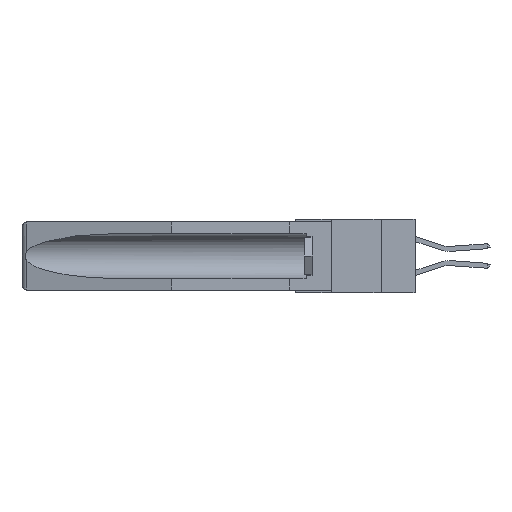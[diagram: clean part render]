
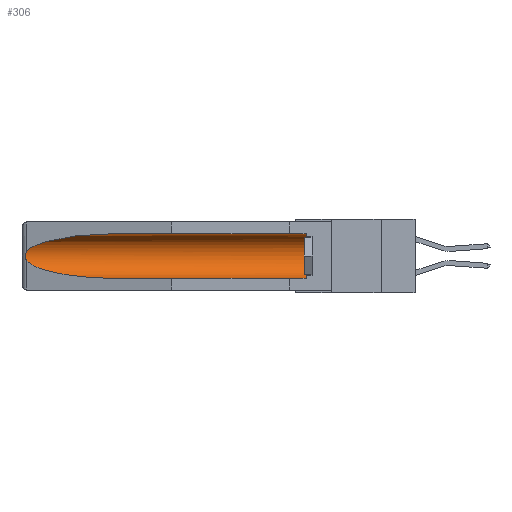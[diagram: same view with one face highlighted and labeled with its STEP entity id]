
A CAD part, left-side view. The second image highlights one B-rep face of the part: STEP entity #306.
In plain terms, the highlighted cylindrical face has radius 2.857 mm (diameter 5.715 mm), a partial arc.
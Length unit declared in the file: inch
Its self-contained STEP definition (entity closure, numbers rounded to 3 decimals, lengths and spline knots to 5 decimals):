
#306 = ADVANCED_FACE ( 'NONE', ( #12683 ), #20967, .F. ) ;
#672 = CARTESIAN_POINT ( 'NONE',  ( 0.26654, 1.53092, -0.15636 ) ) ;
#1336 = CARTESIAN_POINT ( 'NONE',  ( 0.155, 0.126, -0.059 ) ) ;
#1991 = ORIENTED_EDGE ( 'NONE', *, *, #8486, .T. ) ;
#2003 = CARTESIAN_POINT ( 'NONE',  ( 0.155, 0.126, -0.284 ) ) ;
#2503 = CARTESIAN_POINT ( 'NONE',  ( 0.26537, 1.52718, -0.19328 ) ) ;
#3495 = DIRECTION ( 'NONE',  ( 0., 0., 1. ) ) ;
#3614 = CARTESIAN_POINT ( 'NONE',  ( 0.21114, 1.30732, -0.059 ) ) ;
#3765 = DIRECTION ( 'NONE',  ( 0., 1., 0. ) ) ;
#4247 = CARTESIAN_POINT ( 'NONE',  ( 0.26537, 1.52718, -0.19328 ) ) ;
#4786 = VECTOR ( 'NONE', #20074, 39.37008 ) ;
#5399 = CARTESIAN_POINT ( 'NONE',  ( 0.25451, 1.48313, -0.09465 ) ) ;
#5595 = DIRECTION ( 'NONE',  ( 0., 0., 1. ) ) ;
#5802 = EDGE_CURVE ( 'NONE', #7470, #11109, #12739, .T. ) ;
#5821 = CARTESIAN_POINT ( 'NONE',  ( 0.155, -0.30754, -0.059 ) ) ;
#5837 = EDGE_CURVE ( 'NONE', #13670, #10943, #19625, .T. ) ;
#5994 = CARTESIAN_POINT ( 'NONE',  ( 0.21114, 1.30732, -0.284 ) ) ;
#7470 = VERTEX_POINT ( 'NONE', #22293 ) ;
#7852 = CIRCLE ( 'NONE', #11667, 0.1125 ) ;
#7912 = CARTESIAN_POINT ( 'NONE',  ( 0.26655, 1.53094, -0.18657 ) ) ;
#8140 = ORIENTED_EDGE ( 'NONE', *, *, #21844, .T. ) ;
#8207 = EDGE_LOOP ( 'NONE', ( #10516, #8140, #8739, #10500, #1991, #14394 ) ) ;
#8486 = EDGE_CURVE ( 'NONE', #13670, #22188, #7852, .T. ) ;
#8716 = CARTESIAN_POINT ( 'NONE',  ( 0.155, 1.07973, -0.059 ) ) ;
#8739 = ORIENTED_EDGE ( 'NONE', *, *, #15914, .T. ) ;
#9505 = CARTESIAN_POINT ( 'NONE',  ( 0.26537, 1.52718, -0.14972 ) ) ;
#9574 = CARTESIAN_POINT ( 'NONE',  ( 0.2675, 1.53308, -0.17534 ) ) ;
#10500 = ORIENTED_EDGE ( 'NONE', *, *, #5837, .F. ) ;
#10516 = ORIENTED_EDGE ( 'NONE', *, *, #5802, .T. ) ;
#10870 = DIRECTION ( 'NONE',  ( 0., -1., 0. ) ) ;
#10943 = VERTEX_POINT ( 'NONE', #19009 ) ;
#11109 = VERTEX_POINT ( 'NONE', #16170 ) ;
#11667 = AXIS2_PLACEMENT_3D ( 'NONE', #21522, #10870, #5595 ) ;
#11717 =( BOUNDED_CURVE ( )  B_SPLINE_CURVE ( 3, ( #2503, #14869, #5994, #20271 ),
 .UNSPECIFIED., .F., .T. ) 
 B_SPLINE_CURVE_WITH_KNOTS ( ( 4, 4 ),
 ( 0.1948, 1.5708 ),
 .UNSPECIFIED. ) 
 CURVE ( )  GEOMETRIC_REPRESENTATION_ITEM ( )  RATIONAL_B_SPLINE_CURVE ( ( 1., 0.848, 0.848, 1. ) ) 
 REPRESENTATION_ITEM ( '' )  );
#12665 = DIRECTION ( 'NONE',  ( 0., 1., 0. ) ) ;
#12683 = FACE_OUTER_BOUND ( 'NONE', #8207, .T. ) ;
#12739 =( BOUNDED_CURVE ( )  B_SPLINE_CURVE ( 3, ( #8716, #3614, #5399, #21154 ),
 .UNSPECIFIED., .F., .F. ) 
 B_SPLINE_CURVE_WITH_KNOTS ( ( 4, 4 ),
 ( 4.71239, 6.08839 ),
 .UNSPECIFIED. ) 
 CURVE ( )  GEOMETRIC_REPRESENTATION_ITEM ( )  RATIONAL_B_SPLINE_CURVE ( ( 1., 0.848, 0.848, 1. ) ) 
 REPRESENTATION_ITEM ( '' )  );
#13451 = B_SPLINE_CURVE_WITH_KNOTS ( 'NONE', 3,
 ( #9505, #21807, #672, #20219, #20291, #9574, #20052, #7912, #16599, #4247 ),
 .UNSPECIFIED., .F., .F.,
 ( 4, 2, 2, 2, 4 ),
 ( 0., 0.00029, 0.00058, 0.00087, 0.00117 ),
 .UNSPECIFIED. ) ;
#13670 = VERTEX_POINT ( 'NONE', #2003 ) ;
#14394 = ORIENTED_EDGE ( 'NONE', *, *, #18059, .T. ) ;
#14492 = CARTESIAN_POINT ( 'NONE',  ( 0.155, -0.30754, -0.284 ) ) ;
#14869 = CARTESIAN_POINT ( 'NONE',  ( 0.25451, 1.48313, -0.24835 ) ) ;
#15914 = EDGE_CURVE ( 'NONE', #17093, #10943, #11717, .T. ) ;
#16170 = CARTESIAN_POINT ( 'NONE',  ( 0.26537, 1.52718, -0.14972 ) ) ;
#16599 = CARTESIAN_POINT ( 'NONE',  ( 0.26597, 1.5296, -0.19026 ) ) ;
#17088 = AXIS2_PLACEMENT_3D ( 'NONE', #17695, #12665, #3495 ) ;
#17093 = VERTEX_POINT ( 'NONE', #18180 ) ;
#17695 = CARTESIAN_POINT ( 'NONE',  ( 0.155, -0.30754, -0.1715 ) ) ;
#18059 = EDGE_CURVE ( 'NONE', #22188, #7470, #21167, .T. ) ;
#18180 = CARTESIAN_POINT ( 'NONE',  ( 0.26537, 1.52718, -0.19328 ) ) ;
#19009 = CARTESIAN_POINT ( 'NONE',  ( 0.155, 1.07973, -0.284 ) ) ;
#19625 = LINE ( 'NONE', #14492, #22667 ) ;
#20052 = CARTESIAN_POINT ( 'NONE',  ( 0.2673, 1.53269, -0.17917 ) ) ;
#20074 = DIRECTION ( 'NONE',  ( 0., 1., 0. ) ) ;
#20219 = CARTESIAN_POINT ( 'NONE',  ( 0.2673, 1.5327, -0.16383 ) ) ;
#20271 = CARTESIAN_POINT ( 'NONE',  ( 0.155, 1.07973, -0.284 ) ) ;
#20291 = CARTESIAN_POINT ( 'NONE',  ( 0.2675, 1.53308, -0.16763 ) ) ;
#20967 = CYLINDRICAL_SURFACE ( 'NONE', #17088, 0.1125 ) ;
#21154 = CARTESIAN_POINT ( 'NONE',  ( 0.26537, 1.52718, -0.14972 ) ) ;
#21167 = LINE ( 'NONE', #5821, #4786 ) ;
#21522 = CARTESIAN_POINT ( 'NONE',  ( 0.155, 0.126, -0.1715 ) ) ;
#21807 = CARTESIAN_POINT ( 'NONE',  ( 0.26597, 1.52961, -0.15275 ) ) ;
#21844 = EDGE_CURVE ( 'NONE', #11109, #17093, #13451, .T. ) ;
#22188 = VERTEX_POINT ( 'NONE', #1336 ) ;
#22293 = CARTESIAN_POINT ( 'NONE',  ( 0.155, 1.07973, -0.059 ) ) ;
#22667 = VECTOR ( 'NONE', #3765, 39.37008 ) ;
